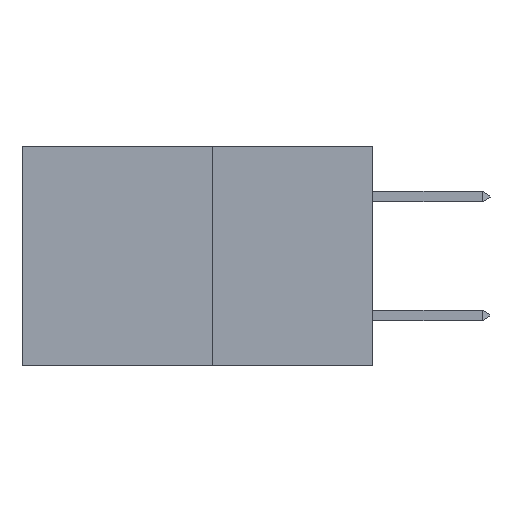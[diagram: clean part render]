
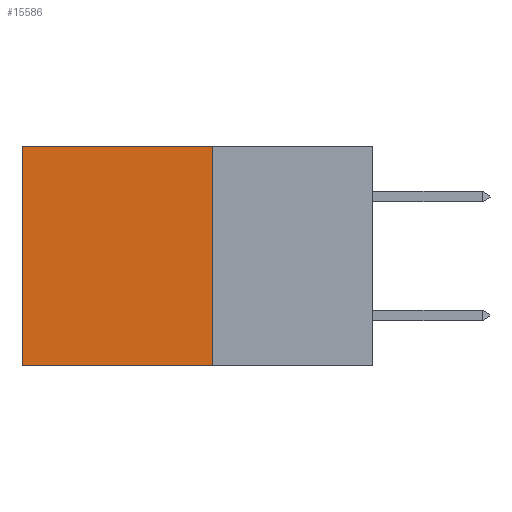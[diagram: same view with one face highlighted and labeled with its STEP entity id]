
A CAD part, left-side view. The second image highlights one B-rep face of the part: STEP entity #15586.
In plain terms, the highlighted planar face has unit normal (-1, 0, 0).
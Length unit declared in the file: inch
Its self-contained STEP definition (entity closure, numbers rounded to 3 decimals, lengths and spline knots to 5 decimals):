
#1484 = EDGE_CURVE ( 'NONE', #12734, #11139, #13509, .T. ) ;
#3261 = ORIENTED_EDGE ( 'NONE', *, *, #3769, .F. ) ;
#3769 = EDGE_CURVE ( 'NONE', #6236, #12734, #4911, .T. ) ;
#3875 = DIRECTION ( 'NONE',  ( 0., 0., -1. ) ) ;
#4035 = VECTOR ( 'NONE', #15645, 39.37008 ) ;
#4438 = VECTOR ( 'NONE', #19238, 39.37008 ) ;
#4911 = LINE ( 'NONE', #16599, #12918 ) ;
#6236 = VERTEX_POINT ( 'NONE', #17445 ) ;
#6623 = EDGE_LOOP ( 'NONE', ( #9478, #11258, #3261, #15693 ) ) ;
#7063 = EDGE_CURVE ( 'NONE', #6236, #14116, #12434, .T. ) ;
#7920 = DIRECTION ( 'NONE',  ( 1., 0., 0. ) ) ;
#8211 = CARTESIAN_POINT ( 'NONE',  ( 0.277, 0.27, 0. ) ) ;
#9478 = ORIENTED_EDGE ( 'NONE', *, *, #16601, .T. ) ;
#9599 = CARTESIAN_POINT ( 'NONE',  ( 0.277, 0.27, -0.37 ) ) ;
#9877 = FACE_OUTER_BOUND ( 'NONE', #6623, .T. ) ;
#11139 = VERTEX_POINT ( 'NONE', #18390 ) ;
#11258 = ORIENTED_EDGE ( 'NONE', *, *, #1484, .F. ) ;
#12434 = LINE ( 'NONE', #8211, #4438 ) ;
#12734 = VERTEX_POINT ( 'NONE', #13052 ) ;
#12918 = VECTOR ( 'NONE', #16535, 39.37008 ) ;
#13052 = CARTESIAN_POINT ( 'NONE',  ( 0.277, 0.27, -0.37 ) ) ;
#13425 = CARTESIAN_POINT ( 'NONE',  ( 0.277, 0.59, -0.37 ) ) ;
#13509 = LINE ( 'NONE', #9599, #4035 ) ;
#13732 = AXIS2_PLACEMENT_3D ( 'NONE', #17412, #7920, #18963 ) ;
#14116 = VERTEX_POINT ( 'NONE', #17972 ) ;
#14273 = PLANE ( 'NONE',  #13732 ) ;
#15586 = ADVANCED_FACE ( 'NONE', ( #9877 ), #14273, .F. ) ;
#15645 = DIRECTION ( 'NONE',  ( 0., 1., 0. ) ) ;
#15693 = ORIENTED_EDGE ( 'NONE', *, *, #7063, .T. ) ;
#16260 = VECTOR ( 'NONE', #3875, 39.37008 ) ;
#16535 = DIRECTION ( 'NONE',  ( 0., 0., -1. ) ) ;
#16599 = CARTESIAN_POINT ( 'NONE',  ( 0.277, 0.27, -0.37 ) ) ;
#16601 = EDGE_CURVE ( 'NONE', #14116, #11139, #19882, .T. ) ;
#17412 = CARTESIAN_POINT ( 'NONE',  ( 0.277, 0.27, -0.37 ) ) ;
#17445 = CARTESIAN_POINT ( 'NONE',  ( 0.277, 0.27, 0. ) ) ;
#17972 = CARTESIAN_POINT ( 'NONE',  ( 0.277, 0.59, 0. ) ) ;
#18390 = CARTESIAN_POINT ( 'NONE',  ( 0.277, 0.59, -0.37 ) ) ;
#18963 = DIRECTION ( 'NONE',  ( 0., 0., -1. ) ) ;
#19238 = DIRECTION ( 'NONE',  ( 0., 1., 0. ) ) ;
#19882 = LINE ( 'NONE', #13425, #16260 ) ;
